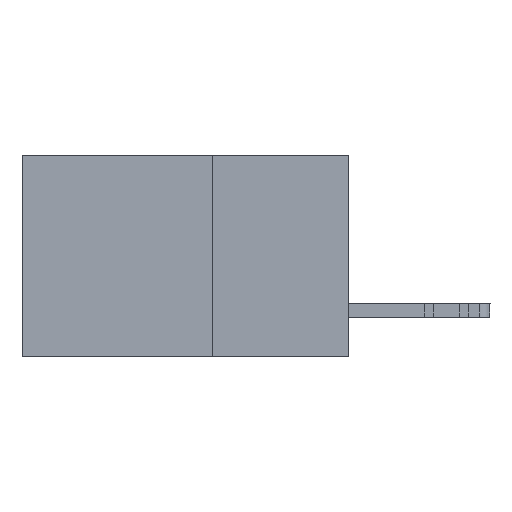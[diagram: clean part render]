
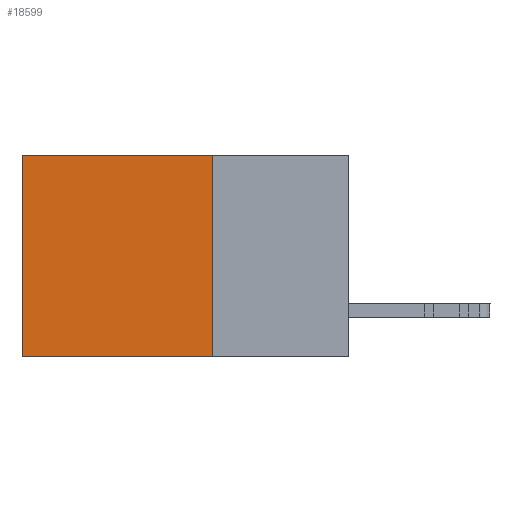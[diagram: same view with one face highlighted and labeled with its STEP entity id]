
A CAD part, left-side view. The second image highlights one B-rep face of the part: STEP entity #18599.
In plain terms, the highlighted planar face has unit normal (-1, 0, 0).
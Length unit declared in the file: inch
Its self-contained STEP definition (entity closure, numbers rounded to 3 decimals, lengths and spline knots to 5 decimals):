
#28 = DIRECTION ( 'NONE',  ( 0., 1., 0. ) ) ;
#1942 = CARTESIAN_POINT ( 'NONE',  ( 0.2615, 0.6, -0.37 ) ) ;
#3739 = VERTEX_POINT ( 'NONE', #21589 ) ;
#5797 = EDGE_CURVE ( 'NONE', #19095, #20593, #17176, .T. ) ;
#6337 = VECTOR ( 'NONE', #28, 39.37008 ) ;
#6968 = AXIS2_PLACEMENT_3D ( 'NONE', #7303, #12231, #12473 ) ;
#7241 = VECTOR ( 'NONE', #16662, 39.37008 ) ;
#7303 = CARTESIAN_POINT ( 'NONE',  ( 0.2615, 0.25, -0.37 ) ) ;
#7952 = EDGE_CURVE ( 'NONE', #22732, #3739, #14006, .T. ) ;
#8371 = ORIENTED_EDGE ( 'NONE', *, *, #7952, .T. ) ;
#10798 = CARTESIAN_POINT ( 'NONE',  ( 0.2615, 0.6, -0.37 ) ) ;
#10880 = LINE ( 'NONE', #1942, #13211 ) ;
#11361 = EDGE_LOOP ( 'NONE', ( #18621, #21014, #21459, #8371 ) ) ;
#12231 = DIRECTION ( 'NONE',  ( 1., 0., 0. ) ) ;
#12473 = DIRECTION ( 'NONE',  ( 0., 0., -1. ) ) ;
#12722 = DIRECTION ( 'NONE',  ( 0., 0., -1. ) ) ;
#12966 = CARTESIAN_POINT ( 'NONE',  ( 0.2615, 0.25, -0.37 ) ) ;
#13211 = VECTOR ( 'NONE', #12722, 39.37008 ) ;
#13514 = EDGE_CURVE ( 'NONE', #22732, #19095, #20006, .T. ) ;
#14006 = LINE ( 'NONE', #18055, #20352 ) ;
#16662 = DIRECTION ( 'NONE',  ( 0., 0., -1. ) ) ;
#16940 = EDGE_CURVE ( 'NONE', #3739, #20593, #10880, .T. ) ;
#17176 = LINE ( 'NONE', #17291, #6337 ) ;
#17291 = CARTESIAN_POINT ( 'NONE',  ( 0.2615, 0.25, -0.37 ) ) ;
#18027 = CARTESIAN_POINT ( 'NONE',  ( 0.2615, 0.25, 0. ) ) ;
#18055 = CARTESIAN_POINT ( 'NONE',  ( 0.2615, 0.25, 0. ) ) ;
#18289 = CARTESIAN_POINT ( 'NONE',  ( 0.2615, 0.25, -0.37 ) ) ;
#18599 = ADVANCED_FACE ( 'NONE', ( #19519 ), #19747, .F. ) ;
#18621 = ORIENTED_EDGE ( 'NONE', *, *, #16940, .T. ) ;
#19095 = VERTEX_POINT ( 'NONE', #12966 ) ;
#19519 = FACE_OUTER_BOUND ( 'NONE', #11361, .T. ) ;
#19747 = PLANE ( 'NONE',  #6968 ) ;
#20006 = LINE ( 'NONE', #18289, #7241 ) ;
#20352 = VECTOR ( 'NONE', #21039, 39.37008 ) ;
#20593 = VERTEX_POINT ( 'NONE', #10798 ) ;
#21014 = ORIENTED_EDGE ( 'NONE', *, *, #5797, .F. ) ;
#21039 = DIRECTION ( 'NONE',  ( 0., 1., 0. ) ) ;
#21459 = ORIENTED_EDGE ( 'NONE', *, *, #13514, .F. ) ;
#21589 = CARTESIAN_POINT ( 'NONE',  ( 0.2615, 0.6, 0. ) ) ;
#22732 = VERTEX_POINT ( 'NONE', #18027 ) ;
